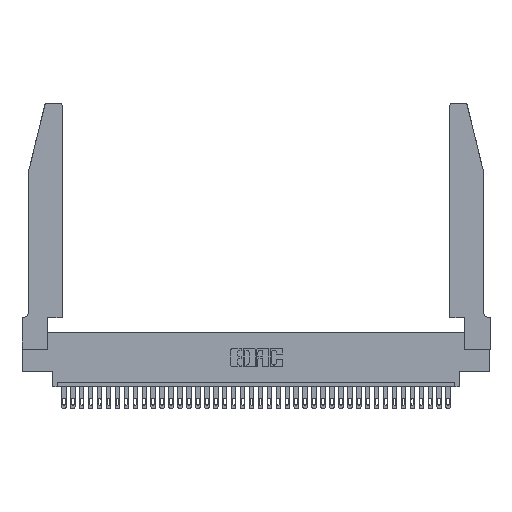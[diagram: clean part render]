
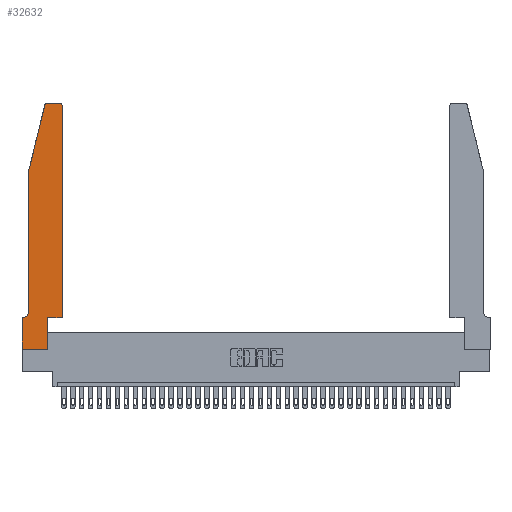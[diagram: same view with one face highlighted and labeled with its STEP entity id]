
A CAD part, top view. The second image highlights one B-rep face of the part: STEP entity #32632.
In plain terms, the highlighted planar face has unit normal (0, 0, 1).
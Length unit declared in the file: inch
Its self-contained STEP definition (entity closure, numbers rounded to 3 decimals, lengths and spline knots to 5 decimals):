
#907 = DIRECTION ( 'NONE',  ( -1., 0., 0. ) ) ;
#1252 = VECTOR ( 'NONE', #14353, 39.37008 ) ;
#1374 = DIRECTION ( 'NONE',  ( 1., 0., 0. ) ) ;
#1833 = ORIENTED_EDGE ( 'NONE', *, *, #11409, .T. ) ;
#1872 = PLANE ( 'NONE',  #15055 ) ;
#1916 = AXIS2_PLACEMENT_3D ( 'NONE', #23756, #20735, #23644 ) ;
#2033 = CARTESIAN_POINT ( 'NONE',  ( 0.2865, 0., 0.37 ) ) ;
#2878 = VERTEX_POINT ( 'NONE', #35147 ) ;
#3270 = LINE ( 'NONE', #28467, #33353 ) ;
#4085 = VERTEX_POINT ( 'NONE', #10827 ) ;
#4210 = ORIENTED_EDGE ( 'NONE', *, *, #20374, .T. ) ;
#4690 = ORIENTED_EDGE ( 'NONE', *, *, #15032, .T. ) ;
#4758 = DIRECTION ( 'NONE',  ( 1., 0., 0. ) ) ;
#4891 = VECTOR ( 'NONE', #23219, 39.37008 ) ;
#5487 = VERTEX_POINT ( 'NONE', #33815 ) ;
#6931 = EDGE_CURVE ( 'NONE', #26398, #9239, #3270, .T. ) ;
#7245 = ORIENTED_EDGE ( 'NONE', *, *, #24269, .T. ) ;
#7282 = EDGE_CURVE ( 'NONE', #12870, #15272, #11333, .T. ) ;
#7307 = CARTESIAN_POINT ( 'NONE',  ( 0., 0.35, 0.37 ) ) ;
#7870 = CARTESIAN_POINT ( 'NONE',  ( 0.2865, 0.35, 0.37 ) ) ;
#8618 = VECTOR ( 'NONE', #9619, 39.37008 ) ;
#9225 = VERTEX_POINT ( 'NONE', #12048 ) ;
#9239 = VERTEX_POINT ( 'NONE', #10669 ) ;
#9242 = VERTEX_POINT ( 'NONE', #31007 ) ;
#9619 = DIRECTION ( 'NONE',  ( 0., -1., 0. ) ) ;
#9627 = EDGE_CURVE ( 'NONE', #19834, #35255, #25689, .T. ) ;
#9663 = CIRCLE ( 'NONE', #22937, 0.07 ) ;
#9879 = LINE ( 'NONE', #33707, #25368 ) ;
#10318 = ORIENTED_EDGE ( 'NONE', *, *, #37651, .T. ) ;
#10669 = CARTESIAN_POINT ( 'NONE',  ( 0.284, 2.75, 0.37 ) ) ;
#10827 = CARTESIAN_POINT ( 'NONE',  ( 0., 0., 0.37 ) ) ;
#11333 = LINE ( 'NONE', #24499, #33570 ) ;
#11409 = EDGE_CURVE ( 'NONE', #5487, #9242, #22384, .T. ) ;
#11629 = DIRECTION ( 'NONE',  ( 0., 0., 1. ) ) ;
#11797 = CARTESIAN_POINT ( 'NONE',  ( 0.4205, 2.75, 0.37 ) ) ;
#12048 = CARTESIAN_POINT ( 'NONE',  ( 0.0755, 0.42, 0.37 ) ) ;
#12369 = CARTESIAN_POINT ( 'NONE',  ( 0., 0.35, 0.37 ) ) ;
#12870 = VERTEX_POINT ( 'NONE', #7870 ) ;
#14353 = DIRECTION ( 'NONE',  ( 1., 0., 0. ) ) ;
#14423 = ORIENTED_EDGE ( 'NONE', *, *, #7282, .T. ) ;
#14762 = VECTOR ( 'NONE', #20808, 39.37008 ) ;
#15000 = ORIENTED_EDGE ( 'NONE', *, *, #23632, .T. ) ;
#15032 = EDGE_CURVE ( 'NONE', #32120, #12870, #9879, .T. ) ;
#15055 = AXIS2_PLACEMENT_3D ( 'NONE', #7307, #27863, #4758 ) ;
#15272 = VERTEX_POINT ( 'NONE', #23355 ) ;
#17339 = CARTESIAN_POINT ( 'NONE',  ( 0., 0., 0.37 ) ) ;
#17672 = EDGE_LOOP ( 'NONE', ( #32263, #28755, #1833, #4210, #7245, #26235, #22899, #10318, #4690, #14423, #21077, #15000 ) ) ;
#18878 = LINE ( 'NONE', #32366, #14762 ) ;
#19834 = VERTEX_POINT ( 'NONE', #27840 ) ;
#20049 = CARTESIAN_POINT ( 'NONE',  ( 0.4205, 2.72, 0.37 ) ) ;
#20098 = EDGE_CURVE ( 'NONE', #9239, #5487, #36056, .T. ) ;
#20374 = EDGE_CURVE ( 'NONE', #9242, #9225, #27689, .T. ) ;
#20735 = DIRECTION ( 'NONE',  ( 0., 0., 1. ) ) ;
#20808 = DIRECTION ( 'NONE',  ( 0., 1., 0. ) ) ;
#21077 = ORIENTED_EDGE ( 'NONE', *, *, #23501, .T. ) ;
#21131 = EDGE_CURVE ( 'NONE', #35255, #4085, #23116, .T. ) ;
#22384 = LINE ( 'NONE', #34786, #30544 ) ;
#22899 = ORIENTED_EDGE ( 'NONE', *, *, #21131, .T. ) ;
#22927 = CARTESIAN_POINT ( 'NONE',  ( 0.0755, 0.35, 0.37 ) ) ;
#22937 = AXIS2_PLACEMENT_3D ( 'NONE', #36095, #26766, #35582 ) ;
#23116 = LINE ( 'NONE', #17339, #4891 ) ;
#23219 = DIRECTION ( 'NONE',  ( 0., -1., 0. ) ) ;
#23355 = CARTESIAN_POINT ( 'NONE',  ( 0.4505, 0.35, 0.37 ) ) ;
#23501 = EDGE_CURVE ( 'NONE', #15272, #2878, #18878, .T. ) ;
#23632 = EDGE_CURVE ( 'NONE', #2878, #26398, #30243, .T. ) ;
#23644 = DIRECTION ( 'NONE',  ( 1., 0., 0. ) ) ;
#23756 = CARTESIAN_POINT ( 'NONE',  ( 0.284, 2.72, 0.37 ) ) ;
#24269 = EDGE_CURVE ( 'NONE', #9225, #19834, #9663, .T. ) ;
#24499 = CARTESIAN_POINT ( 'NONE',  ( 0.4505, 0.35, 0.37 ) ) ;
#25368 = VECTOR ( 'NONE', #30629, 39.37008 ) ;
#25689 = LINE ( 'NONE', #22927, #36153 ) ;
#26235 = ORIENTED_EDGE ( 'NONE', *, *, #9627, .T. ) ;
#26398 = VERTEX_POINT ( 'NONE', #11797 ) ;
#26766 = DIRECTION ( 'NONE',  ( 0., 0., -1. ) ) ;
#26803 = FACE_OUTER_BOUND ( 'NONE', #17672, .T. ) ;
#27137 = LINE ( 'NONE', #37491, #1252 ) ;
#27689 = LINE ( 'NONE', #33405, #8618 ) ;
#27840 = CARTESIAN_POINT ( 'NONE',  ( 0.0055, 0.35, 0.37 ) ) ;
#27863 = DIRECTION ( 'NONE',  ( 0., 0., 1. ) ) ;
#28467 = CARTESIAN_POINT ( 'NONE',  ( 0.2605, 2.75, 0.37 ) ) ;
#28755 = ORIENTED_EDGE ( 'NONE', *, *, #20098, .T. ) ;
#28983 = AXIS2_PLACEMENT_3D ( 'NONE', #20049, #11629, #37441 ) ;
#30243 = CIRCLE ( 'NONE', #28983, 0.03 ) ;
#30544 = VECTOR ( 'NONE', #35904, 39.37008 ) ;
#30629 = DIRECTION ( 'NONE',  ( 0., 1., 0. ) ) ;
#31007 = CARTESIAN_POINT ( 'NONE',  ( 0.0755, 2., 0.37 ) ) ;
#32120 = VERTEX_POINT ( 'NONE', #2033 ) ;
#32263 = ORIENTED_EDGE ( 'NONE', *, *, #6931, .T. ) ;
#32366 = CARTESIAN_POINT ( 'NONE',  ( 0.4505, 0.35, 0.37 ) ) ;
#32632 = ADVANCED_FACE ( 'NONE', ( #26803 ), #1872, .T. ) ;
#33353 = VECTOR ( 'NONE', #37263, 39.37008 ) ;
#33405 = CARTESIAN_POINT ( 'NONE',  ( 0.0755, 2., 0.37 ) ) ;
#33570 = VECTOR ( 'NONE', #1374, 39.37008 ) ;
#33707 = CARTESIAN_POINT ( 'NONE',  ( 0.2865, 0.35, 0.37 ) ) ;
#33815 = CARTESIAN_POINT ( 'NONE',  ( 0.25487, 2.72718, 0.37 ) ) ;
#34786 = CARTESIAN_POINT ( 'NONE',  ( 0.0755, 2., 0.37 ) ) ;
#35147 = CARTESIAN_POINT ( 'NONE',  ( 0.4505, 2.72, 0.37 ) ) ;
#35255 = VERTEX_POINT ( 'NONE', #12369 ) ;
#35582 = DIRECTION ( 'NONE',  ( -1., 0., 0. ) ) ;
#35904 = DIRECTION ( 'NONE',  ( -0.239, -0.971, 0. ) ) ;
#36056 = CIRCLE ( 'NONE', #1916, 0.03 ) ;
#36095 = CARTESIAN_POINT ( 'NONE',  ( 0.0055, 0.42, 0.37 ) ) ;
#36153 = VECTOR ( 'NONE', #907, 39.37008 ) ;
#37263 = DIRECTION ( 'NONE',  ( -1., 0., 0. ) ) ;
#37441 = DIRECTION ( 'NONE',  ( 1., 0., 0. ) ) ;
#37491 = CARTESIAN_POINT ( 'NONE',  ( 0., 0., 0.37 ) ) ;
#37651 = EDGE_CURVE ( 'NONE', #4085, #32120, #27137, .T. ) ;
